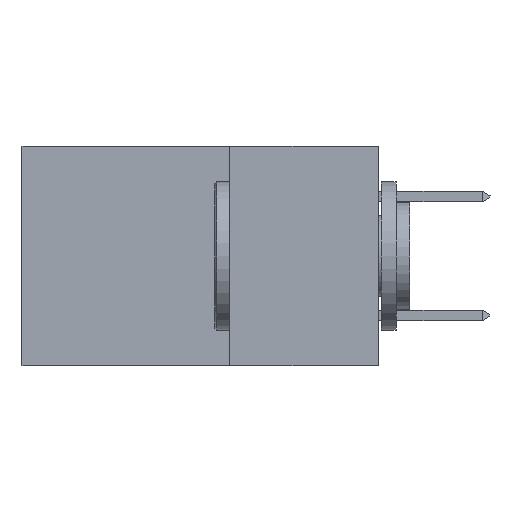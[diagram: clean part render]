
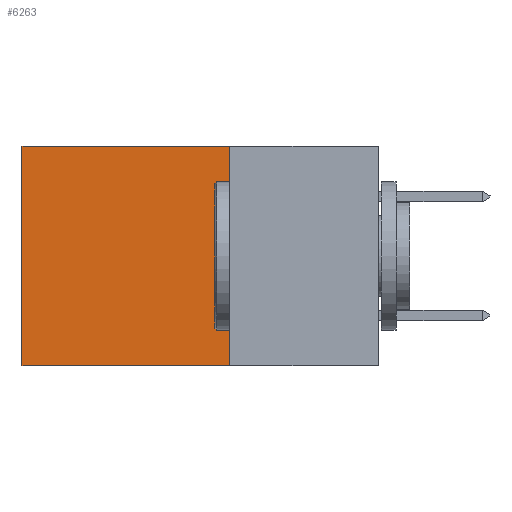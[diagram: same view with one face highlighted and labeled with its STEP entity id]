
A CAD part, left-side view. The second image highlights one B-rep face of the part: STEP entity #6263.
In plain terms, the highlighted planar face has unit normal (-1, 0, 0).
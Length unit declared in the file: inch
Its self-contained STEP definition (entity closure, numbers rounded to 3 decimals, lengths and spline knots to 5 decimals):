
#143 = LINE ( 'NONE', #15775, #6727 ) ;
#372 = LINE ( 'NONE', #12975, #11985 ) ;
#993 = CARTESIAN_POINT ( 'NONE',  ( 0.2615, 0.25, 0. ) ) ;
#1115 = DIRECTION ( 'NONE',  ( 0., 1., 0. ) ) ;
#1267 = AXIS2_PLACEMENT_3D ( 'NONE', #3681, #8937, #2213 ) ;
#1718 = CARTESIAN_POINT ( 'NONE',  ( 0.2615, 0.6, 0. ) ) ;
#1937 = VERTEX_POINT ( 'NONE', #1718 ) ;
#2083 = CARTESIAN_POINT ( 'NONE',  ( 0.2615, 0.25, -0.37 ) ) ;
#2213 = DIRECTION ( 'NONE',  ( 0., 0., -1. ) ) ;
#2451 = ORIENTED_EDGE ( 'NONE', *, *, #8783, .F. ) ;
#2521 = ORIENTED_EDGE ( 'NONE', *, *, #5496, .T. ) ;
#2780 = EDGE_CURVE ( 'NONE', #5097, #1937, #4002, .T. ) ;
#2939 = VECTOR ( 'NONE', #12122, 39.37008 ) ;
#3418 = EDGE_LOOP ( 'NONE', ( #2521, #2451, #14239, #13306 ) ) ;
#3681 = CARTESIAN_POINT ( 'NONE',  ( 0.2615, 0.25, -0.37 ) ) ;
#4002 = LINE ( 'NONE', #993, #10244 ) ;
#5097 = VERTEX_POINT ( 'NONE', #6521 ) ;
#5496 = EDGE_CURVE ( 'NONE', #1937, #8389, #143, .T. ) ;
#5938 = CARTESIAN_POINT ( 'NONE',  ( 0.2615, 0.25, -0.37 ) ) ;
#6235 = DIRECTION ( 'NONE',  ( 0., 1., 0. ) ) ;
#6263 = ADVANCED_FACE ( 'NONE', ( #10124 ), #15496, .F. ) ;
#6521 = CARTESIAN_POINT ( 'NONE',  ( 0.2615, 0.25, 0. ) ) ;
#6727 = VECTOR ( 'NONE', #14554, 39.37008 ) ;
#8182 = LINE ( 'NONE', #5938, #2939 ) ;
#8389 = VERTEX_POINT ( 'NONE', #12077 ) ;
#8783 = EDGE_CURVE ( 'NONE', #9790, #8389, #372, .T. ) ;
#8937 = DIRECTION ( 'NONE',  ( 1., 0., 0. ) ) ;
#9579 = EDGE_CURVE ( 'NONE', #5097, #9790, #8182, .T. ) ;
#9790 = VERTEX_POINT ( 'NONE', #2083 ) ;
#10124 = FACE_OUTER_BOUND ( 'NONE', #3418, .T. ) ;
#10244 = VECTOR ( 'NONE', #6235, 39.37008 ) ;
#11985 = VECTOR ( 'NONE', #1115, 39.37008 ) ;
#12077 = CARTESIAN_POINT ( 'NONE',  ( 0.2615, 0.6, -0.37 ) ) ;
#12122 = DIRECTION ( 'NONE',  ( 0., 0., -1. ) ) ;
#12975 = CARTESIAN_POINT ( 'NONE',  ( 0.2615, 0.25, -0.37 ) ) ;
#13306 = ORIENTED_EDGE ( 'NONE', *, *, #2780, .T. ) ;
#14239 = ORIENTED_EDGE ( 'NONE', *, *, #9579, .F. ) ;
#14554 = DIRECTION ( 'NONE',  ( 0., 0., -1. ) ) ;
#15496 = PLANE ( 'NONE',  #1267 ) ;
#15775 = CARTESIAN_POINT ( 'NONE',  ( 0.2615, 0.6, -0.37 ) ) ;
